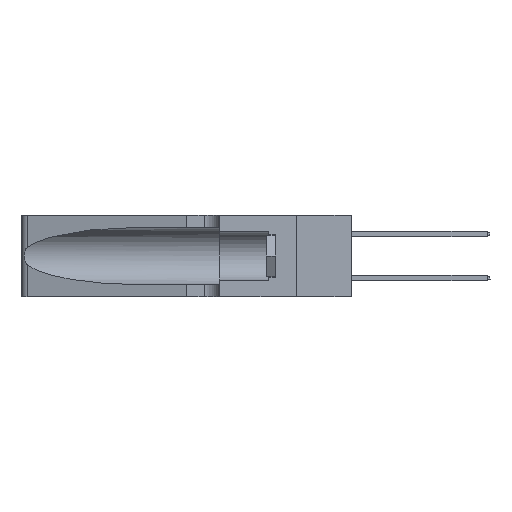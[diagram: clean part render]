
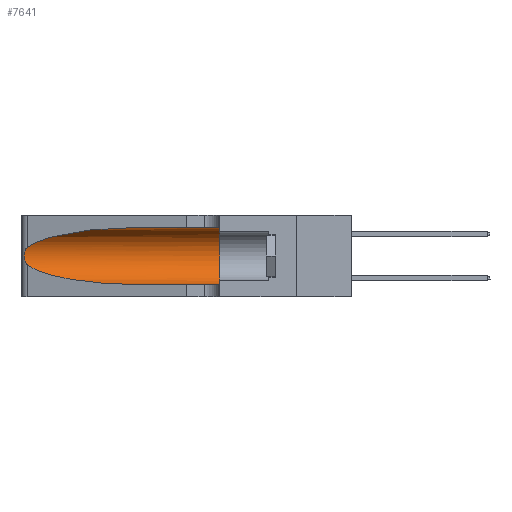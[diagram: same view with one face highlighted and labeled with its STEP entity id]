
A CAD part, left-side view. The second image highlights one B-rep face of the part: STEP entity #7641.
In plain terms, the highlighted cylindrical face has radius 3.308 mm (diameter 6.617 mm), a partial arc.
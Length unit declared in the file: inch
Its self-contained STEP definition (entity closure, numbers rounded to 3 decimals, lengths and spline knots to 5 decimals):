
#1101 = CARTESIAN_POINT ( 'NONE',  ( 0.25854, 1.2359, 0.20912 ) ) ;
#1656 = CARTESIAN_POINT ( 'NONE',  ( 0.1305, 0.35, 0.05475 ) ) ;
#1845 = VERTEX_POINT ( 'NONE', #32655 ) ;
#2225 = CARTESIAN_POINT ( 'NONE',  ( 0.1305, 0.72297, 0.05475 ) ) ;
#2394 = VERTEX_POINT ( 'NONE', #1656 ) ;
#4031 = CARTESIAN_POINT ( 'NONE',  ( 0.25789, 1.23486, 0.15765 ) ) ;
#4306 = CARTESIAN_POINT ( 'NONE',  ( 0.1305, 1.61858, 0.05475 ) ) ;
#4584 = ORIENTED_EDGE ( 'NONE', *, *, #13887, .F. ) ;
#5510 = ORIENTED_EDGE ( 'NONE', *, *, #29258, .T. ) ;
#5676 = CARTESIAN_POINT ( 'NONE',  ( 0.25487, 1.22718, 0.22369 ) ) ;
#6426 = VECTOR ( 'NONE', #28215, 39.37008 ) ;
#7064 = VECTOR ( 'NONE', #25184, 39.37008 ) ;
#7419 = VERTEX_POINT ( 'NONE', #28257 ) ;
#7641 = ADVANCED_FACE ( 'NONE', ( #9406 ), #27341, .F. ) ;
#7878 = ORIENTED_EDGE ( 'NONE', *, *, #23589, .T. ) ;
#8629 = CARTESIAN_POINT ( 'NONE',  ( 0.1305, 0.35, 0.185 ) ) ;
#9034 =( BOUNDED_CURVE ( )  B_SPLINE_CURVE ( 3, ( #13397, #18773, #24037, #31419 ),
 .UNSPECIFIED., .F., .F. ) 
 B_SPLINE_CURVE_WITH_KNOTS ( ( 4, 4 ),
 ( 1.5708, 2.84003 ),
 .UNSPECIFIED. ) 
 CURVE ( )  GEOMETRIC_REPRESENTATION_ITEM ( )  RATIONAL_B_SPLINE_CURVE ( ( 1., 0.87, 0.87, 1. ) ) 
 REPRESENTATION_ITEM ( '' )  );
#9386 = ORIENTED_EDGE ( 'NONE', *, *, #21680, .T. ) ;
#9406 = FACE_OUTER_BOUND ( 'NONE', #16351, .T. ) ;
#9603 = ORIENTED_EDGE ( 'NONE', *, *, #24960, .T. ) ;
#11056 = ORIENTED_EDGE ( 'NONE', *, *, #30371, .F. ) ;
#11606 = CARTESIAN_POINT ( 'NONE',  ( 0.25639, 1.23184, 0.21858 ) ) ;
#11751 = CARTESIAN_POINT ( 'NONE',  ( 0.25487, 1.22718, 0.14631 ) ) ;
#11836 = CARTESIAN_POINT ( 'NONE',  ( 0.25856, 1.23593, 0.16098 ) ) ;
#12052 = CIRCLE ( 'NONE', #13722, 0.13025 ) ;
#12053 = B_SPLINE_CURVE_WITH_KNOTS ( 'NONE', 3,
 ( #5676, #16662, #11606, #25393, #1101, #28038, #14657, #25025, #27557, #11836, #4031, #12071, #32994, #19788 ),
 .UNSPECIFIED., .F., .F.,
 ( 4, 2, 2, 2, 2, 2, 4 ),
 ( 0., 0.00027, 0.00053, 0.00107, 0.0016, 0.00187, 0.00214 ),
 .UNSPECIFIED. ) ;
#12071 = CARTESIAN_POINT ( 'NONE',  ( 0.25639, 1.23186, 0.15144 ) ) ;
#13397 = CARTESIAN_POINT ( 'NONE',  ( 0.1305, 0.72297, 0.31525 ) ) ;
#13722 = AXIS2_PLACEMENT_3D ( 'NONE', #8629, #29601, #16355 ) ;
#13887 = EDGE_CURVE ( 'NONE', #1845, #33139, #24611, .T. ) ;
#14657 = CARTESIAN_POINT ( 'NONE',  ( 0.26075, 1.23896, 0.19203 ) ) ;
#16351 = EDGE_LOOP ( 'NONE', ( #5510, #9386, #9603, #7878, #11056, #4584 ) ) ;
#16355 = DIRECTION ( 'NONE',  ( 0., 0., 1. ) ) ;
#16662 = CARTESIAN_POINT ( 'NONE',  ( 0.25555, 1.22994, 0.2215 ) ) ;
#18072 = CARTESIAN_POINT ( 'NONE',  ( 0.1305, 1.61858, 0.185 ) ) ;
#18241 = CARTESIAN_POINT ( 'NONE',  ( 0.2373, 1.15595, 0.08982 ) ) ;
#18773 = CARTESIAN_POINT ( 'NONE',  ( 0.18966, 0.96281, 0.31525 ) ) ;
#19042 = CARTESIAN_POINT ( 'NONE',  ( 0.1305, 0.35, 0.31525 ) ) ;
#19788 = CARTESIAN_POINT ( 'NONE',  ( 0.25487, 1.22718, 0.14631 ) ) ;
#20607 = LINE ( 'NONE', #4306, #6426 ) ;
#21386 = AXIS2_PLACEMENT_3D ( 'NONE', #18072, #34415, #26556 ) ;
#21680 = EDGE_CURVE ( 'NONE', #7419, #32260, #12053, .T. ) ;
#23589 = EDGE_CURVE ( 'NONE', #26058, #2394, #20607, .T. ) ;
#24037 = CARTESIAN_POINT ( 'NONE',  ( 0.2373, 1.15595, 0.28018 ) ) ;
#24611 = LINE ( 'NONE', #33585, #7064 ) ;
#24960 = EDGE_CURVE ( 'NONE', #32260, #26058, #34181, .T. ) ;
#25025 = CARTESIAN_POINT ( 'NONE',  ( 0.26075, 1.23896, 0.178 ) ) ;
#25184 = DIRECTION ( 'NONE',  ( 0., -1., 0. ) ) ;
#25393 = CARTESIAN_POINT ( 'NONE',  ( 0.25787, 1.23484, 0.2124 ) ) ;
#26058 = VERTEX_POINT ( 'NONE', #28065 ) ;
#26268 = CARTESIAN_POINT ( 'NONE',  ( 0.18966, 0.96281, 0.05475 ) ) ;
#26556 = DIRECTION ( 'NONE',  ( 0., 0., -1. ) ) ;
#27341 = CYLINDRICAL_SURFACE ( 'NONE', #21386, 0.13025 ) ;
#27557 = CARTESIAN_POINT ( 'NONE',  ( 0.26017, 1.23833, 0.17102 ) ) ;
#28038 = CARTESIAN_POINT ( 'NONE',  ( 0.26018, 1.23835, 0.19895 ) ) ;
#28065 = CARTESIAN_POINT ( 'NONE',  ( 0.1305, 0.72297, 0.05475 ) ) ;
#28215 = DIRECTION ( 'NONE',  ( 0., -1., 0. ) ) ;
#28257 = CARTESIAN_POINT ( 'NONE',  ( 0.25487, 1.22718, 0.22369 ) ) ;
#29258 = EDGE_CURVE ( 'NONE', #1845, #7419, #9034, .T. ) ;
#29601 = DIRECTION ( 'NONE',  ( 0., 1., 0. ) ) ;
#30371 = EDGE_CURVE ( 'NONE', #33139, #2394, #12052, .T. ) ;
#31419 = CARTESIAN_POINT ( 'NONE',  ( 0.25487, 1.22718, 0.22369 ) ) ;
#32260 = VERTEX_POINT ( 'NONE', #11751 ) ;
#32655 = CARTESIAN_POINT ( 'NONE',  ( 0.1305, 0.72297, 0.31525 ) ) ;
#32994 = CARTESIAN_POINT ( 'NONE',  ( 0.25555, 1.22993, 0.14849 ) ) ;
#33139 = VERTEX_POINT ( 'NONE', #19042 ) ;
#33428 = CARTESIAN_POINT ( 'NONE',  ( 0.25487, 1.22718, 0.14631 ) ) ;
#33585 = CARTESIAN_POINT ( 'NONE',  ( 0.1305, 1.61858, 0.31525 ) ) ;
#34181 =( BOUNDED_CURVE ( )  B_SPLINE_CURVE ( 3, ( #33428, #18241, #26268, #2225 ),
 .UNSPECIFIED., .F., .F. ) 
 B_SPLINE_CURVE_WITH_KNOTS ( ( 4, 4 ),
 ( 3.44316, 4.71239 ),
 .UNSPECIFIED. ) 
 CURVE ( )  GEOMETRIC_REPRESENTATION_ITEM ( )  RATIONAL_B_SPLINE_CURVE ( ( 1., 0.87, 0.87, 1. ) ) 
 REPRESENTATION_ITEM ( '' )  );
#34415 = DIRECTION ( 'NONE',  ( 0., -1., 0. ) ) ;
